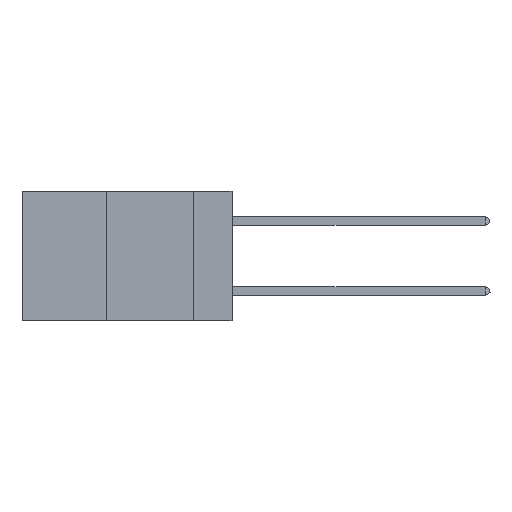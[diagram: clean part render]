
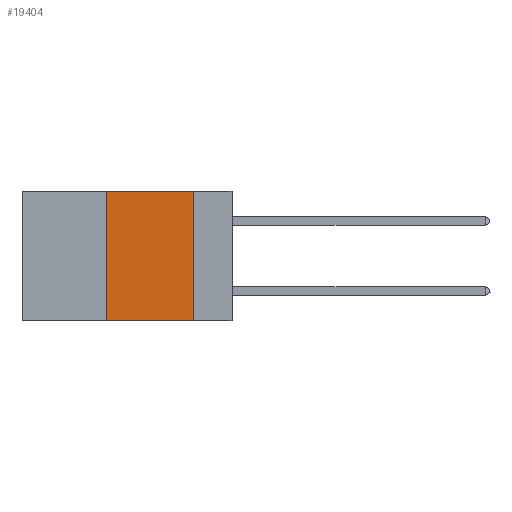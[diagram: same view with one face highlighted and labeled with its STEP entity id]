
A CAD part, left-side view. The second image highlights one B-rep face of the part: STEP entity #19404.
In plain terms, the highlighted planar face has unit normal (-1, 0, 0).
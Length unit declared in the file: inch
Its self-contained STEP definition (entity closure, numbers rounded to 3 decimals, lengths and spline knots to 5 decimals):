
#104 = DIRECTION ( 'NONE',  ( 0., -1., 0. ) ) ;
#2347 = LINE ( 'NONE', #21129, #25911 ) ;
#4541 = CARTESIAN_POINT ( 'NONE',  ( 0., 0.11, -0.37 ) ) ;
#5995 = VERTEX_POINT ( 'NONE', #13094 ) ;
#6072 = EDGE_CURVE ( 'NONE', #25898, #19484, #13261, .T. ) ;
#6318 = ORIENTED_EDGE ( 'NONE', *, *, #30224, .F. ) ;
#7878 = CARTESIAN_POINT ( 'NONE',  ( 0., 0.6, 0. ) ) ;
#9626 = DIRECTION ( 'NONE',  ( 0., 0., -1. ) ) ;
#10795 = ORIENTED_EDGE ( 'NONE', *, *, #14650, .F. ) ;
#11735 = CARTESIAN_POINT ( 'NONE',  ( 0., 0.36, 0. ) ) ;
#12635 = ORIENTED_EDGE ( 'NONE', *, *, #19618, .F. ) ;
#13030 = CARTESIAN_POINT ( 'NONE',  ( 0., 0.36, 0. ) ) ;
#13094 = CARTESIAN_POINT ( 'NONE',  ( 0., 0.11, 0. ) ) ;
#13261 = LINE ( 'NONE', #21346, #34609 ) ;
#13703 = VECTOR ( 'NONE', #15740, 39.37008 ) ;
#14650 = EDGE_CURVE ( 'NONE', #5995, #19484, #2347, .T. ) ;
#15740 = DIRECTION ( 'NONE',  ( 0., -1., 0. ) ) ;
#18390 = LINE ( 'NONE', #7878, #13703 ) ;
#19172 = VERTEX_POINT ( 'NONE', #13030 ) ;
#19341 = AXIS2_PLACEMENT_3D ( 'NONE', #33299, #20505, #9626 ) ;
#19404 = ADVANCED_FACE ( 'NONE', ( #28560 ), #20328, .F. ) ;
#19484 = VERTEX_POINT ( 'NONE', #4541 ) ;
#19618 = EDGE_CURVE ( 'NONE', #19172, #5995, #18390, .T. ) ;
#20328 = PLANE ( 'NONE',  #19341 ) ;
#20505 = DIRECTION ( 'NONE',  ( 1., 0., 0. ) ) ;
#21129 = CARTESIAN_POINT ( 'NONE',  ( 0., 0.11, 0. ) ) ;
#21346 = CARTESIAN_POINT ( 'NONE',  ( 0., 0.6, -0.37 ) ) ;
#23914 = VECTOR ( 'NONE', #27858, 39.37008 ) ;
#25071 = LINE ( 'NONE', #11735, #23914 ) ;
#25898 = VERTEX_POINT ( 'NONE', #26514 ) ;
#25911 = VECTOR ( 'NONE', #31802, 39.37008 ) ;
#26514 = CARTESIAN_POINT ( 'NONE',  ( 0., 0.36, -0.37 ) ) ;
#27858 = DIRECTION ( 'NONE',  ( 0., 0., 1. ) ) ;
#28560 = FACE_OUTER_BOUND ( 'NONE', #30271, .T. ) ;
#30224 = EDGE_CURVE ( 'NONE', #25898, #19172, #25071, .T. ) ;
#30271 = EDGE_LOOP ( 'NONE', ( #10795, #12635, #6318, #31805 ) ) ;
#31802 = DIRECTION ( 'NONE',  ( 0., 0., -1. ) ) ;
#31805 = ORIENTED_EDGE ( 'NONE', *, *, #6072, .T. ) ;
#33299 = CARTESIAN_POINT ( 'NONE',  ( 0., 0.6, 0. ) ) ;
#34609 = VECTOR ( 'NONE', #104, 39.37008 ) ;
